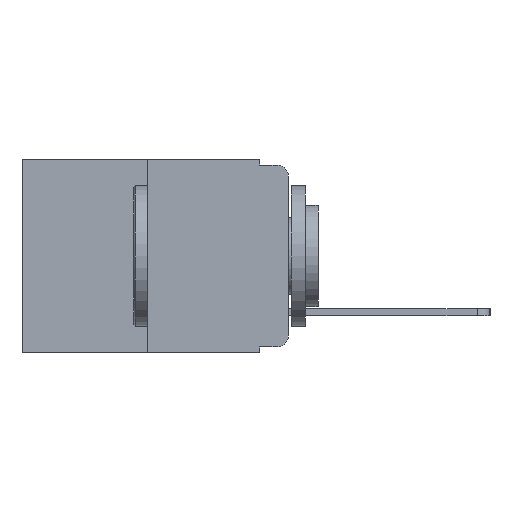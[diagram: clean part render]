
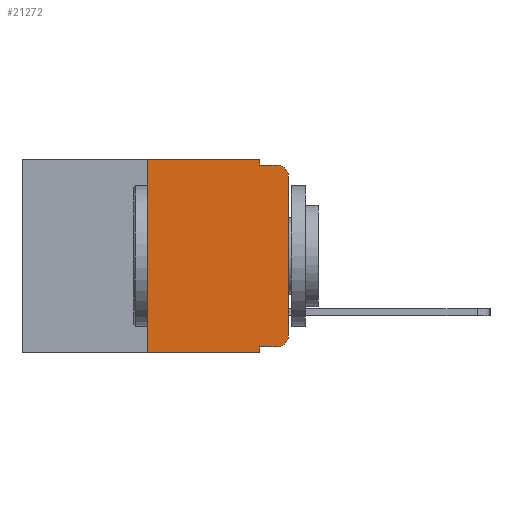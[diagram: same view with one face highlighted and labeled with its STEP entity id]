
A CAD part, left-side view. The second image highlights one B-rep face of the part: STEP entity #21272.
In plain terms, the highlighted planar face has unit normal (-1, 0, 0).
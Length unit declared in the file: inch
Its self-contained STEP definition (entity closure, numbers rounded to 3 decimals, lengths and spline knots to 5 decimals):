
#66 = ORIENTED_EDGE ( 'NONE', *, *, #11543, .T. ) ;
#287 = VECTOR ( 'NONE', #19529, 39.37008 ) ;
#296 = ORIENTED_EDGE ( 'NONE', *, *, #19182, .F. ) ;
#864 = ORIENTED_EDGE ( 'NONE', *, *, #18126, .F. ) ;
#1037 = EDGE_CURVE ( 'NONE', #3577, #9169, #7775, .T. ) ;
#1059 = CARTESIAN_POINT ( 'NONE',  ( 0., 0., 0. ) ) ;
#1199 = LINE ( 'NONE', #14894, #5127 ) ;
#1537 = AXIS2_PLACEMENT_3D ( 'NONE', #19480, #9729, #21088 ) ;
#1687 = VERTEX_POINT ( 'NONE', #9433 ) ;
#1947 = ORIENTED_EDGE ( 'NONE', *, *, #13233, .F. ) ;
#2136 = ORIENTED_EDGE ( 'NONE', *, *, #15948, .F. ) ;
#2181 = ORIENTED_EDGE ( 'NONE', *, *, #8546, .T. ) ;
#2297 = VERTEX_POINT ( 'NONE', #5829 ) ;
#3325 = CARTESIAN_POINT ( 'NONE',  ( 0., 0., -0.03 ) ) ;
#3466 = CARTESIAN_POINT ( 'NONE',  ( 0., 0.051, -0.01 ) ) ;
#3472 = CARTESIAN_POINT ( 'NONE',  ( 0., 0.25, 0. ) ) ;
#3519 = VERTEX_POINT ( 'NONE', #16290 ) ;
#3577 = VERTEX_POINT ( 'NONE', #19030 ) ;
#3747 = ORIENTED_EDGE ( 'NONE', *, *, #14864, .F. ) ;
#4339 = AXIS2_PLACEMENT_3D ( 'NONE', #8363, #19753, #9999 ) ;
#4407 = CARTESIAN_POINT ( 'NONE',  ( 0., 0.25, 0. ) ) ;
#4514 = VECTOR ( 'NONE', #11689, 39.37008 ) ;
#4841 = DIRECTION ( 'NONE',  ( 0., -1., 0. ) ) ;
#4939 = DIRECTION ( 'NONE',  ( 0., 0., 1. ) ) ;
#5109 = LINE ( 'NONE', #4407, #17803 ) ;
#5127 = VECTOR ( 'NONE', #18159, 39.37008 ) ;
#5569 = EDGE_LOOP ( 'NONE', ( #13721, #14493, #296, #864, #1947, #2136, #2181, #3747, #10654, #66 ) ) ;
#5829 = CARTESIAN_POINT ( 'NONE',  ( 0., 0.02, -0.333 ) ) ;
#5958 = VERTEX_POINT ( 'NONE', #6236 ) ;
#6135 = DIRECTION ( 'NONE',  ( 0., 0., 1. ) ) ;
#6236 = CARTESIAN_POINT ( 'NONE',  ( 0., 0.02, -0.01 ) ) ;
#7588 = FACE_OUTER_BOUND ( 'NONE', #5569, .T. ) ;
#7775 = LINE ( 'NONE', #1059, #20279 ) ;
#7990 = LINE ( 'NONE', #13192, #11850 ) ;
#8363 = CARTESIAN_POINT ( 'NONE',  ( 0., 0.02, -0.313 ) ) ;
#8546 = EDGE_CURVE ( 'NONE', #3519, #16000, #13130, .T. ) ;
#9061 = LINE ( 'NONE', #10956, #4514 ) ;
#9169 = VERTEX_POINT ( 'NONE', #3325 ) ;
#9433 = CARTESIAN_POINT ( 'NONE',  ( 0., 0.051, -0.333 ) ) ;
#9729 = DIRECTION ( 'NONE',  ( -1., 0., 0. ) ) ;
#9731 = LINE ( 'NONE', #11552, #13608 ) ;
#9999 = DIRECTION ( 'NONE',  ( 0., 0., -1. ) ) ;
#10046 = VECTOR ( 'NONE', #16872, 39.37008 ) ;
#10628 = CIRCLE ( 'NONE', #4339, 0.02 ) ;
#10654 = ORIENTED_EDGE ( 'NONE', *, *, #13775, .T. ) ;
#10688 = CARTESIAN_POINT ( 'NONE',  ( 0., 0.051, 0. ) ) ;
#10772 = DIRECTION ( 'NONE',  ( 0., 0., -1. ) ) ;
#10956 = CARTESIAN_POINT ( 'NONE',  ( 0., 0.473, 0. ) ) ;
#11004 = VERTEX_POINT ( 'NONE', #3466 ) ;
#11427 = CARTESIAN_POINT ( 'NONE',  ( 0., 0.473, -0.343 ) ) ;
#11512 = AXIS2_PLACEMENT_3D ( 'NONE', #18893, #20495, #10772 ) ;
#11543 = EDGE_CURVE ( 'NONE', #2297, #3577, #10628, .T. ) ;
#11552 = CARTESIAN_POINT ( 'NONE',  ( 0., 0.051, -0.01 ) ) ;
#11689 = DIRECTION ( 'NONE',  ( 0., -1., 0. ) ) ;
#11850 = VECTOR ( 'NONE', #4841, 39.37008 ) ;
#13130 = LINE ( 'NONE', #11427, #287 ) ;
#13192 = CARTESIAN_POINT ( 'NONE',  ( 0., 0.051, -0.333 ) ) ;
#13223 = DIRECTION ( 'NONE',  ( 0., -1., 0. ) ) ;
#13233 = EDGE_CURVE ( 'NONE', #18727, #15763, #9061, .T. ) ;
#13608 = VECTOR ( 'NONE', #13223, 39.37008 ) ;
#13721 = ORIENTED_EDGE ( 'NONE', *, *, #1037, .T. ) ;
#13775 = EDGE_CURVE ( 'NONE', #1687, #2297, #7990, .T. ) ;
#14493 = ORIENTED_EDGE ( 'NONE', *, *, #20260, .T. ) ;
#14864 = EDGE_CURVE ( 'NONE', #1687, #16000, #1199, .T. ) ;
#14894 = CARTESIAN_POINT ( 'NONE',  ( 0., 0.051, 0. ) ) ;
#15233 = CARTESIAN_POINT ( 'NONE',  ( 0., 0.051, 0. ) ) ;
#15763 = VERTEX_POINT ( 'NONE', #10688 ) ;
#15948 = EDGE_CURVE ( 'NONE', #3519, #18727, #5109, .T. ) ;
#16000 = VERTEX_POINT ( 'NONE', #19419 ) ;
#16290 = CARTESIAN_POINT ( 'NONE',  ( 0., 0.25, -0.343 ) ) ;
#16872 = DIRECTION ( 'NONE',  ( 0., 0., -1. ) ) ;
#17281 = PLANE ( 'NONE',  #11512 ) ;
#17620 = CIRCLE ( 'NONE', #1537, 0.02 ) ;
#17803 = VECTOR ( 'NONE', #6135, 39.37008 ) ;
#18126 = EDGE_CURVE ( 'NONE', #15763, #11004, #18731, .T. ) ;
#18159 = DIRECTION ( 'NONE',  ( 0., 0., -1. ) ) ;
#18727 = VERTEX_POINT ( 'NONE', #3472 ) ;
#18731 = LINE ( 'NONE', #15233, #10046 ) ;
#18893 = CARTESIAN_POINT ( 'NONE',  ( 0., 0.473, 0. ) ) ;
#19030 = CARTESIAN_POINT ( 'NONE',  ( 0., 0., -0.313 ) ) ;
#19182 = EDGE_CURVE ( 'NONE', #11004, #5958, #9731, .T. ) ;
#19419 = CARTESIAN_POINT ( 'NONE',  ( 0., 0.051, -0.343 ) ) ;
#19480 = CARTESIAN_POINT ( 'NONE',  ( 0., 0.02, -0.03 ) ) ;
#19529 = DIRECTION ( 'NONE',  ( 0., -1., 0. ) ) ;
#19753 = DIRECTION ( 'NONE',  ( -1., 0., 0. ) ) ;
#20260 = EDGE_CURVE ( 'NONE', #9169, #5958, #17620, .T. ) ;
#20279 = VECTOR ( 'NONE', #4939, 39.37008 ) ;
#20495 = DIRECTION ( 'NONE',  ( 1., 0., 0. ) ) ;
#21088 = DIRECTION ( 'NONE',  ( 0., 0., -1. ) ) ;
#21272 = ADVANCED_FACE ( 'NONE', ( #7588 ), #17281, .F. ) ;
